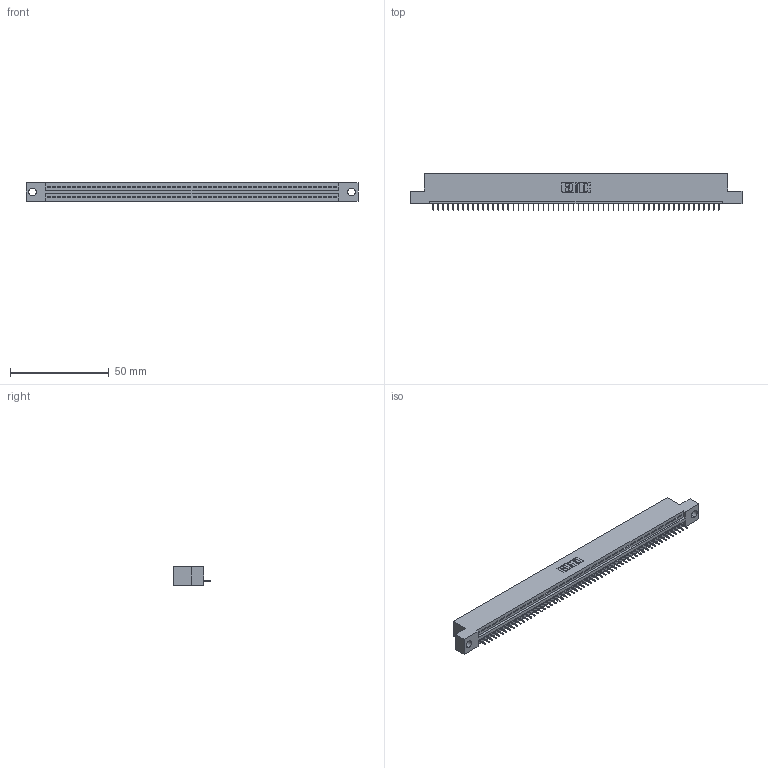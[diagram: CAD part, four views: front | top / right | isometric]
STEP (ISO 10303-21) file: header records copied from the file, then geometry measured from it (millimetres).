
FILE_DESCRIPTION (( 'STEP AP203' ), '1' );
FILE_NAME ('395-058-525-104.STEP', '2020-09-24T18:22:53', ( '' ), ( '' ), 'SwSTEP 2.0', 'SolidWorks 2020', '' );
FILE_SCHEMA (( 'CONFIG_CONTROL_DESIGN' ));
Length unit declared in the file: inch
Products named in the file (3): 395-058-525-104; 345-292-001_345-293-125; 345 Part_Flush Mounting Lugs - 0.156 Dia-TH
Assembly tree (59 placements, depth 2):
  395-058-525-104
    345 Part_Flush Mounting Lugs - 0.156 Dia-TH
    345-292-001_345-293-125  x58
Bounding box: 168.53 x 18.72 x 9.4 mm (x, y, z)
Volume: 15813.5 mm3; surface area: 20251.2 mm2
Topology: 59 solids, 59 shells, 3722 faces, 10781 edges, 6954 vertices
Faces by surface type: plane 2748, cylinder 974
Entity records: 41575 total; most frequent: CARTESIAN_POINT 7206, ORIENTED_EDGE 7198, DIRECTION 6271, EDGE_CURVE 3599, LINE 3239, VECTOR 3239, VERTEX_POINT 2394, AXIS2_PLACEMENT_3D 1516
